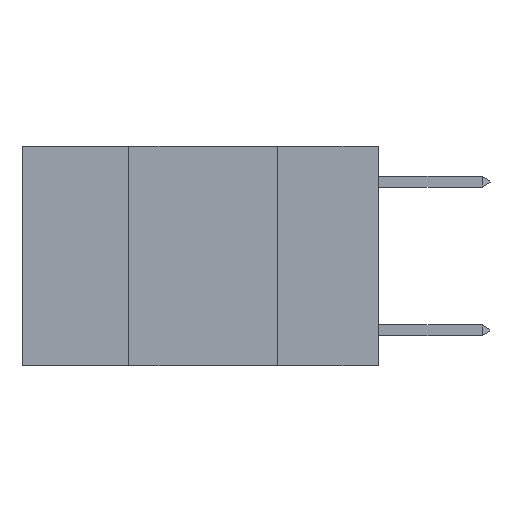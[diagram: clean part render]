
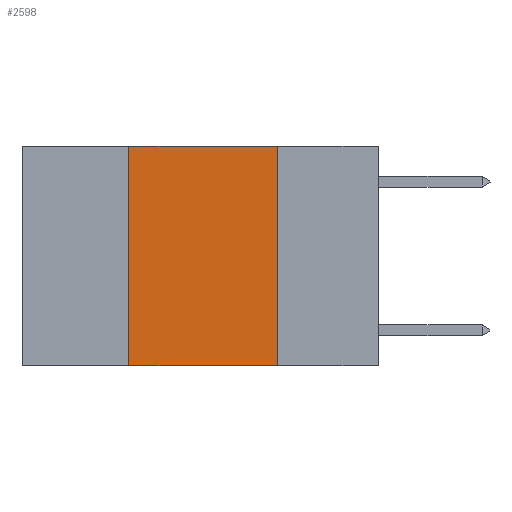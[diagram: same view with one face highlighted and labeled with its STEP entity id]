
A CAD part, left-side view. The second image highlights one B-rep face of the part: STEP entity #2598.
In plain terms, the highlighted planar face has unit normal (-1, 0, 0).
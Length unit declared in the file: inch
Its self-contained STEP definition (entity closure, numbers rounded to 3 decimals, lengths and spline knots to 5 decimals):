
#424 = DIRECTION ( 'NONE',  ( 0., -1., 0. ) ) ;
#563 = FACE_OUTER_BOUND ( 'NONE', #2667, .T. ) ;
#949 = DIRECTION ( 'NONE',  ( 0., 0., -1. ) ) ;
#1354 = VERTEX_POINT ( 'NONE', #8978 ) ;
#1467 = AXIS2_PLACEMENT_3D ( 'NONE', #2720, #6323, #949 ) ;
#1962 = CARTESIAN_POINT ( 'NONE',  ( 0., 0.6, 0. ) ) ;
#2598 = ADVANCED_FACE ( 'NONE', ( #563 ), #8834, .F. ) ;
#2664 = VERTEX_POINT ( 'NONE', #2847 ) ;
#2667 = EDGE_LOOP ( 'NONE', ( #10249, #4218, #9872, #9316 ) ) ;
#2720 = CARTESIAN_POINT ( 'NONE',  ( 0., 0.6, 0. ) ) ;
#2847 = CARTESIAN_POINT ( 'NONE',  ( 0., 0.42, -0.37 ) ) ;
#3796 = DIRECTION ( 'NONE',  ( 0., -1., 0. ) ) ;
#3973 = LINE ( 'NONE', #7567, #10515 ) ;
#4218 = ORIENTED_EDGE ( 'NONE', *, *, #11004, .F. ) ;
#4493 = EDGE_CURVE ( 'NONE', #7107, #10940, #7118, .T. ) ;
#4541 = CARTESIAN_POINT ( 'NONE',  ( 0., 0.42, 0. ) ) ;
#4804 = LINE ( 'NONE', #4541, #5103 ) ;
#4924 = EDGE_CURVE ( 'NONE', #2664, #1354, #4804, .T. ) ;
#5103 = VECTOR ( 'NONE', #11316, 39.37008 ) ;
#5711 = EDGE_CURVE ( 'NONE', #2664, #10940, #3973, .T. ) ;
#5745 = DIRECTION ( 'NONE',  ( 0., 0., -1. ) ) ;
#6323 = DIRECTION ( 'NONE',  ( 1., 0., 0. ) ) ;
#7067 = VECTOR ( 'NONE', #3796, 39.37008 ) ;
#7107 = VERTEX_POINT ( 'NONE', #10290 ) ;
#7118 = LINE ( 'NONE', #10767, #11299 ) ;
#7567 = CARTESIAN_POINT ( 'NONE',  ( 0., 0.6, -0.37 ) ) ;
#8834 = PLANE ( 'NONE',  #1467 ) ;
#8978 = CARTESIAN_POINT ( 'NONE',  ( 0., 0.42, 0. ) ) ;
#9313 = LINE ( 'NONE', #1962, #7067 ) ;
#9316 = ORIENTED_EDGE ( 'NONE', *, *, #5711, .T. ) ;
#9872 = ORIENTED_EDGE ( 'NONE', *, *, #4924, .F. ) ;
#10249 = ORIENTED_EDGE ( 'NONE', *, *, #4493, .F. ) ;
#10290 = CARTESIAN_POINT ( 'NONE',  ( 0., 0.17, 0. ) ) ;
#10515 = VECTOR ( 'NONE', #424, 39.37008 ) ;
#10767 = CARTESIAN_POINT ( 'NONE',  ( 0., 0.17, 0. ) ) ;
#10940 = VERTEX_POINT ( 'NONE', #11330 ) ;
#11004 = EDGE_CURVE ( 'NONE', #1354, #7107, #9313, .T. ) ;
#11299 = VECTOR ( 'NONE', #5745, 39.37008 ) ;
#11316 = DIRECTION ( 'NONE',  ( 0., 0., 1. ) ) ;
#11330 = CARTESIAN_POINT ( 'NONE',  ( 0., 0.17, -0.37 ) ) ;
